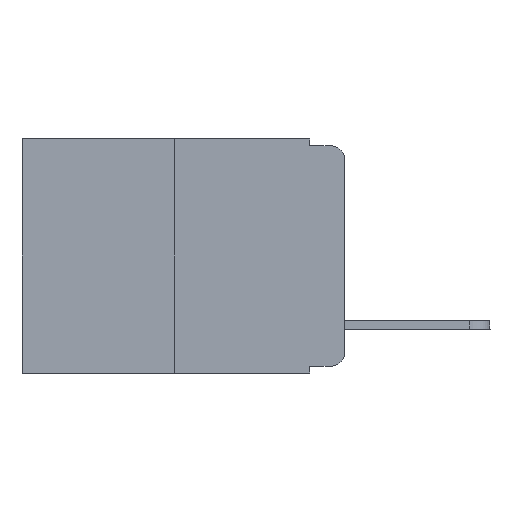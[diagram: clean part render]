
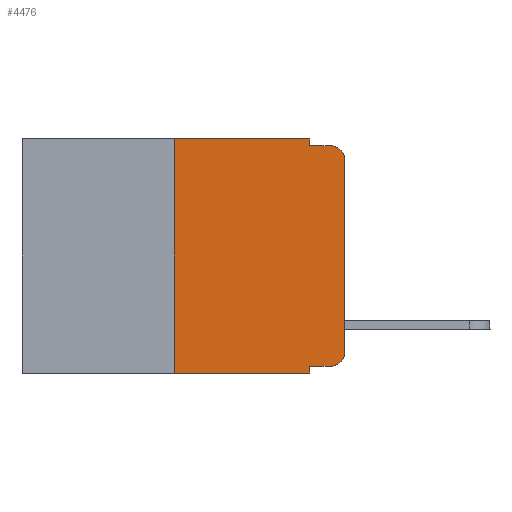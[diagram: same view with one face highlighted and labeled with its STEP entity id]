
A CAD part, left-side view. The second image highlights one B-rep face of the part: STEP entity #4476.
In plain terms, the highlighted planar face has unit normal (-1, 0, 0).
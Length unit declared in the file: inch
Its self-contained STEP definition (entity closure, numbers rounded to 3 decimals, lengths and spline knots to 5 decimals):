
#442 = CARTESIAN_POINT ( 'NONE',  ( 0., 0.051, -0.01 ) ) ;
#798 = LINE ( 'NONE', #17212, #4544 ) ;
#979 = CARTESIAN_POINT ( 'NONE',  ( 0., 0.051, 0. ) ) ;
#1085 = CARTESIAN_POINT ( 'NONE',  ( 0., 0.473, -0.343 ) ) ;
#1108 = CARTESIAN_POINT ( 'NONE',  ( 0., 0.25, 0. ) ) ;
#1208 = CARTESIAN_POINT ( 'NONE',  ( 0., 0.02, -0.01 ) ) ;
#1666 = ORIENTED_EDGE ( 'NONE', *, *, #7295, .T. ) ;
#1728 = ORIENTED_EDGE ( 'NONE', *, *, #10086, .F. ) ;
#1919 = DIRECTION ( 'NONE',  ( 0., 0., -1. ) ) ;
#1965 = VERTEX_POINT ( 'NONE', #13311 ) ;
#2070 = VERTEX_POINT ( 'NONE', #1208 ) ;
#2619 = CARTESIAN_POINT ( 'NONE',  ( 0., 0., 0. ) ) ;
#2867 = VERTEX_POINT ( 'NONE', #5008 ) ;
#3179 = EDGE_CURVE ( 'NONE', #11602, #1965, #798, .T. ) ;
#3484 = VERTEX_POINT ( 'NONE', #12973 ) ;
#3833 = LINE ( 'NONE', #15953, #13489 ) ;
#3897 = CARTESIAN_POINT ( 'NONE',  ( 0., 0.25, -0.343 ) ) ;
#4006 = DIRECTION ( 'NONE',  ( 0., 0., -1. ) ) ;
#4344 = VECTOR ( 'NONE', #10549, 39.37008 ) ;
#4468 = DIRECTION ( 'NONE',  ( 0., -1., 0. ) ) ;
#4476 = ADVANCED_FACE ( 'NONE', ( #13530 ), #5257, .F. ) ;
#4544 = VECTOR ( 'NONE', #8793, 39.37008 ) ;
#4792 = DIRECTION ( 'NONE',  ( -1., 0., 0. ) ) ;
#5008 = CARTESIAN_POINT ( 'NONE',  ( 0., 0., -0.313 ) ) ;
#5257 = PLANE ( 'NONE',  #6210 ) ;
#5330 = CIRCLE ( 'NONE', #13062, 0.02 ) ;
#5639 = CARTESIAN_POINT ( 'NONE',  ( 0., 0.473, 0. ) ) ;
#5649 = LINE ( 'NONE', #11311, #15410 ) ;
#6210 = AXIS2_PLACEMENT_3D ( 'NONE', #5639, #14944, #6429 ) ;
#6221 = ORIENTED_EDGE ( 'NONE', *, *, #10276, .F. ) ;
#6332 = VERTEX_POINT ( 'NONE', #442 ) ;
#6368 = DIRECTION ( 'NONE',  ( 0., -1., 0. ) ) ;
#6429 = DIRECTION ( 'NONE',  ( 0., 0., -1. ) ) ;
#6510 = DIRECTION ( 'NONE',  ( 0., 0., -1. ) ) ;
#7126 = EDGE_CURVE ( 'NONE', #1965, #2867, #11357, .T. ) ;
#7200 = CARTESIAN_POINT ( 'NONE',  ( 0., 0.051, 0. ) ) ;
#7295 = EDGE_CURVE ( 'NONE', #10444, #2070, #5330, .T. ) ;
#7815 = DIRECTION ( 'NONE',  ( 0., -1., 0. ) ) ;
#8274 = VERTEX_POINT ( 'NONE', #3897 ) ;
#8667 = EDGE_CURVE ( 'NONE', #2867, #10444, #9216, .T. ) ;
#8793 = DIRECTION ( 'NONE',  ( 0., -1., 0. ) ) ;
#9214 = ORIENTED_EDGE ( 'NONE', *, *, #11904, .F. ) ;
#9215 = EDGE_CURVE ( 'NONE', #6332, #2070, #3833, .T. ) ;
#9216 = LINE ( 'NONE', #2619, #12619 ) ;
#9274 = ORIENTED_EDGE ( 'NONE', *, *, #7126, .T. ) ;
#9351 = ORIENTED_EDGE ( 'NONE', *, *, #8667, .T. ) ;
#9912 = LINE ( 'NONE', #7200, #16957 ) ;
#10042 = ORIENTED_EDGE ( 'NONE', *, *, #10547, .T. ) ;
#10086 = EDGE_CURVE ( 'NONE', #8274, #3484, #13391, .T. ) ;
#10276 = EDGE_CURVE ( 'NONE', #11602, #14035, #9912, .T. ) ;
#10444 = VERTEX_POINT ( 'NONE', #10701 ) ;
#10547 = EDGE_CURVE ( 'NONE', #8274, #14035, #17671, .T. ) ;
#10549 = DIRECTION ( 'NONE',  ( 0., 0., 1. ) ) ;
#10561 = VERTEX_POINT ( 'NONE', #979 ) ;
#10701 = CARTESIAN_POINT ( 'NONE',  ( 0., 0., -0.03 ) ) ;
#11159 = ORIENTED_EDGE ( 'NONE', *, *, #14209, .F. ) ;
#11311 = CARTESIAN_POINT ( 'NONE',  ( 0., 0.473, 0. ) ) ;
#11357 = CIRCLE ( 'NONE', #13076, 0.02 ) ;
#11602 = VERTEX_POINT ( 'NONE', #11777 ) ;
#11641 = VECTOR ( 'NONE', #4006, 39.37008 ) ;
#11665 = EDGE_LOOP ( 'NONE', ( #9351, #1666, #14797, #11159, #9214, #1728, #10042, #6221, #14967, #9274 ) ) ;
#11777 = CARTESIAN_POINT ( 'NONE',  ( 0., 0.051, -0.333 ) ) ;
#11904 = EDGE_CURVE ( 'NONE', #3484, #10561, #5649, .T. ) ;
#12619 = VECTOR ( 'NONE', #13225, 39.37008 ) ;
#12714 = CARTESIAN_POINT ( 'NONE',  ( 0., 0.051, -0.343 ) ) ;
#12973 = CARTESIAN_POINT ( 'NONE',  ( 0., 0.25, 0. ) ) ;
#13062 = AXIS2_PLACEMENT_3D ( 'NONE', #17085, #4792, #1919 ) ;
#13076 = AXIS2_PLACEMENT_3D ( 'NONE', #16016, #14588, #6510 ) ;
#13225 = DIRECTION ( 'NONE',  ( 0., 0., 1. ) ) ;
#13311 = CARTESIAN_POINT ( 'NONE',  ( 0., 0.02, -0.333 ) ) ;
#13369 = VECTOR ( 'NONE', #7815, 39.37008 ) ;
#13391 = LINE ( 'NONE', #1108, #4344 ) ;
#13489 = VECTOR ( 'NONE', #6368, 39.37008 ) ;
#13530 = FACE_OUTER_BOUND ( 'NONE', #11665, .T. ) ;
#13598 = CARTESIAN_POINT ( 'NONE',  ( 0., 0.051, 0. ) ) ;
#14035 = VERTEX_POINT ( 'NONE', #12714 ) ;
#14209 = EDGE_CURVE ( 'NONE', #10561, #6332, #16193, .T. ) ;
#14588 = DIRECTION ( 'NONE',  ( -1., 0., 0. ) ) ;
#14797 = ORIENTED_EDGE ( 'NONE', *, *, #9215, .F. ) ;
#14944 = DIRECTION ( 'NONE',  ( 1., 0., 0. ) ) ;
#14967 = ORIENTED_EDGE ( 'NONE', *, *, #3179, .T. ) ;
#15333 = DIRECTION ( 'NONE',  ( 0., 0., -1. ) ) ;
#15410 = VECTOR ( 'NONE', #4468, 39.37008 ) ;
#15953 = CARTESIAN_POINT ( 'NONE',  ( 0., 0.051, -0.01 ) ) ;
#16016 = CARTESIAN_POINT ( 'NONE',  ( 0., 0.02, -0.313 ) ) ;
#16193 = LINE ( 'NONE', #13598, #11641 ) ;
#16957 = VECTOR ( 'NONE', #15333, 39.37008 ) ;
#17085 = CARTESIAN_POINT ( 'NONE',  ( 0., 0.02, -0.03 ) ) ;
#17212 = CARTESIAN_POINT ( 'NONE',  ( 0., 0.051, -0.333 ) ) ;
#17671 = LINE ( 'NONE', #1085, #13369 ) ;
